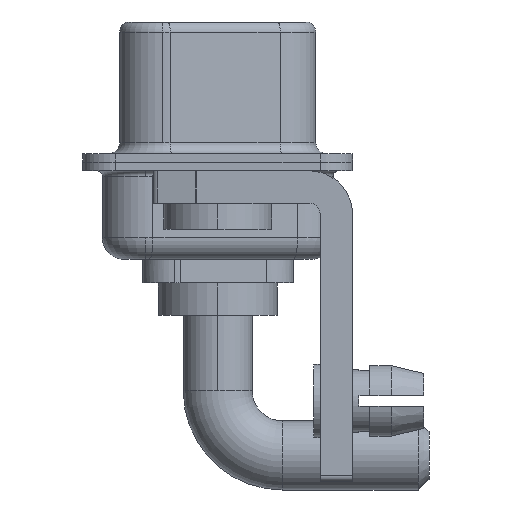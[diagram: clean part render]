
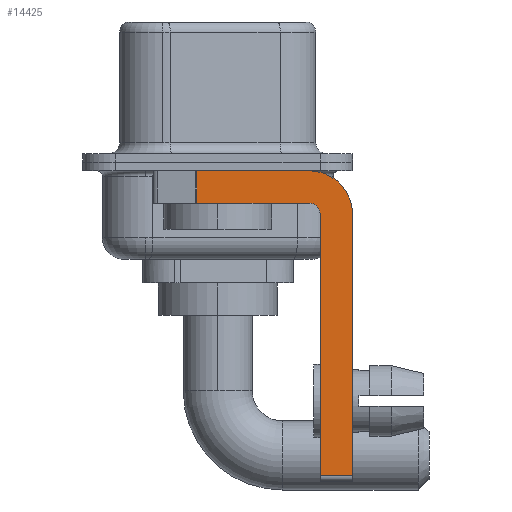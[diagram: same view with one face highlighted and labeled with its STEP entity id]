
A CAD part, left-side view. The second image highlights one B-rep face of the part: STEP entity #14425.
In plain terms, the highlighted planar face has unit normal (-1, 0, 0).
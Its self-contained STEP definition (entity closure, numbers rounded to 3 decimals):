
#82 = CARTESIAN_POINT ( 'NONE',  ( -2.9, 0.978, -1.9 ) ) ;
#185 = CARTESIAN_POINT ( 'NONE',  ( -2.9, -6.25, -2.4 ) ) ;
#775 = CIRCLE ( 'NONE', #12550, 2. ) ;
#814 = EDGE_CURVE ( 'NONE', #1396, #5618, #13986, .T. ) ;
#1002 = CARTESIAN_POINT ( 'NONE',  ( -2.9, 0.978, -1.9 ) ) ;
#1086 = LINE ( 'NONE', #1002, #1631 ) ;
#1117 = EDGE_CURVE ( 'NONE', #5618, #12890, #4486, .T. ) ;
#1396 = VERTEX_POINT ( 'NONE', #12146 ) ;
#1447 = DIRECTION ( 'NONE',  ( 1., 0., 0. ) ) ;
#1513 = VECTOR ( 'NONE', #5352, 1000. ) ;
#1631 = VECTOR ( 'NONE', #7675, 1000. ) ;
#1938 = VERTEX_POINT ( 'NONE', #82 ) ;
#1945 = CARTESIAN_POINT ( 'NONE',  ( -2.9, -4.25, -2.4 ) ) ;
#2116 = LINE ( 'NONE', #5173, #1513 ) ;
#2155 = EDGE_CURVE ( 'NONE', #12890, #1938, #2116, .T. ) ;
#2533 = VECTOR ( 'NONE', #4742, 1000. ) ;
#2982 = DIRECTION ( 'NONE',  ( 0., 0., -1. ) ) ;
#3042 = LINE ( 'NONE', #8256, #2533 ) ;
#3240 = CARTESIAN_POINT ( 'NONE',  ( -2.9, 0.978, -0.4 ) ) ;
#3259 = CARTESIAN_POINT ( 'NONE',  ( -2.9, -4.25, -0.4 ) ) ;
#3373 = LINE ( 'NONE', #7389, #6664 ) ;
#3714 = CARTESIAN_POINT ( 'NONE',  ( -2.9, -4.75, -2.4 ) ) ;
#4331 = LINE ( 'NONE', #9536, #9041 ) ;
#4486 = CIRCLE ( 'NONE', #14688, 0.5 ) ;
#4742 = DIRECTION ( 'NONE',  ( 0., -1., 0. ) ) ;
#5173 = CARTESIAN_POINT ( 'NONE',  ( -2.9, -4.25, -1.9 ) ) ;
#5352 = DIRECTION ( 'NONE',  ( 0., 1., 0. ) ) ;
#5464 = EDGE_LOOP ( 'NONE', ( #13384, #10273, #10235, #12625, #14656, #7921, #7833, #16026 ) ) ;
#5618 = VERTEX_POINT ( 'NONE', #3714 ) ;
#5724 = EDGE_CURVE ( 'NONE', #6297, #10072, #3373, .T. ) ;
#6032 = CARTESIAN_POINT ( 'NONE',  ( -2.9, -4.25, -1.9 ) ) ;
#6097 = AXIS2_PLACEMENT_3D ( 'NONE', #13569, #6877, #14522 ) ;
#6297 = VERTEX_POINT ( 'NONE', #185 ) ;
#6439 = VECTOR ( 'NONE', #11484, 1000. ) ;
#6664 = VECTOR ( 'NONE', #12644, 1000. ) ;
#6877 = DIRECTION ( 'NONE',  ( 1., 0., 0. ) ) ;
#6996 = EDGE_CURVE ( 'NONE', #8666, #10044, #4331, .T. ) ;
#7374 = EDGE_CURVE ( 'NONE', #8666, #1938, #1086, .T. ) ;
#7389 = CARTESIAN_POINT ( 'NONE',  ( -2.9, -6.25, -2.4 ) ) ;
#7675 = DIRECTION ( 'NONE',  ( 0., 0., -1. ) ) ;
#7833 = ORIENTED_EDGE ( 'NONE', *, *, #5724, .F. ) ;
#7921 = ORIENTED_EDGE ( 'NONE', *, *, #12845, .T. ) ;
#8038 = CARTESIAN_POINT ( 'NONE',  ( -2.9, -4.25, -2.4 ) ) ;
#8256 = CARTESIAN_POINT ( 'NONE',  ( -2.9, -4.25, -14.55 ) ) ;
#8391 = EDGE_CURVE ( 'NONE', #10044, #6297, #775, .T. ) ;
#8666 = VERTEX_POINT ( 'NONE', #3240 ) ;
#9041 = VECTOR ( 'NONE', #14814, 1000. ) ;
#9536 = CARTESIAN_POINT ( 'NONE',  ( -2.9, 3., -0.4 ) ) ;
#10044 = VERTEX_POINT ( 'NONE', #3259 ) ;
#10072 = VERTEX_POINT ( 'NONE', #15988 ) ;
#10235 = ORIENTED_EDGE ( 'NONE', *, *, #2155, .F. ) ;
#10273 = ORIENTED_EDGE ( 'NONE', *, *, #7374, .T. ) ;
#10638 = FACE_OUTER_BOUND ( 'NONE', #5464, .T. ) ;
#11181 = DIRECTION ( 'NONE',  ( 0., 0., 1. ) ) ;
#11484 = DIRECTION ( 'NONE',  ( 0., 0., 1. ) ) ;
#11568 = CARTESIAN_POINT ( 'NONE',  ( -2.9, -4.75, -14.8 ) ) ;
#12117 = PLANE ( 'NONE',  #6097 ) ;
#12146 = CARTESIAN_POINT ( 'NONE',  ( -2.9, -4.75, -14.55 ) ) ;
#12550 = AXIS2_PLACEMENT_3D ( 'NONE', #8038, #1447, #2982 ) ;
#12625 = ORIENTED_EDGE ( 'NONE', *, *, #1117, .F. ) ;
#12644 = DIRECTION ( 'NONE',  ( 0., 0., -1. ) ) ;
#12845 = EDGE_CURVE ( 'NONE', #1396, #10072, #3042, .T. ) ;
#12890 = VERTEX_POINT ( 'NONE', #6032 ) ;
#13384 = ORIENTED_EDGE ( 'NONE', *, *, #6996, .F. ) ;
#13569 = CARTESIAN_POINT ( 'NONE',  ( -2.9, -4.25, -2.4 ) ) ;
#13986 = LINE ( 'NONE', #11568, #6439 ) ;
#14425 = ADVANCED_FACE ( 'NONE', ( #10638 ), #12117, .F. ) ;
#14522 = DIRECTION ( 'NONE',  ( 0., 0., -1. ) ) ;
#14656 = ORIENTED_EDGE ( 'NONE', *, *, #814, .F. ) ;
#14688 = AXIS2_PLACEMENT_3D ( 'NONE', #1945, #16714, #11181 ) ;
#14814 = DIRECTION ( 'NONE',  ( 0., -1., 0. ) ) ;
#15988 = CARTESIAN_POINT ( 'NONE',  ( -2.9, -6.25, -14.55 ) ) ;
#16026 = ORIENTED_EDGE ( 'NONE', *, *, #8391, .F. ) ;
#16714 = DIRECTION ( 'NONE',  ( -1., 0., 0. ) ) ;
